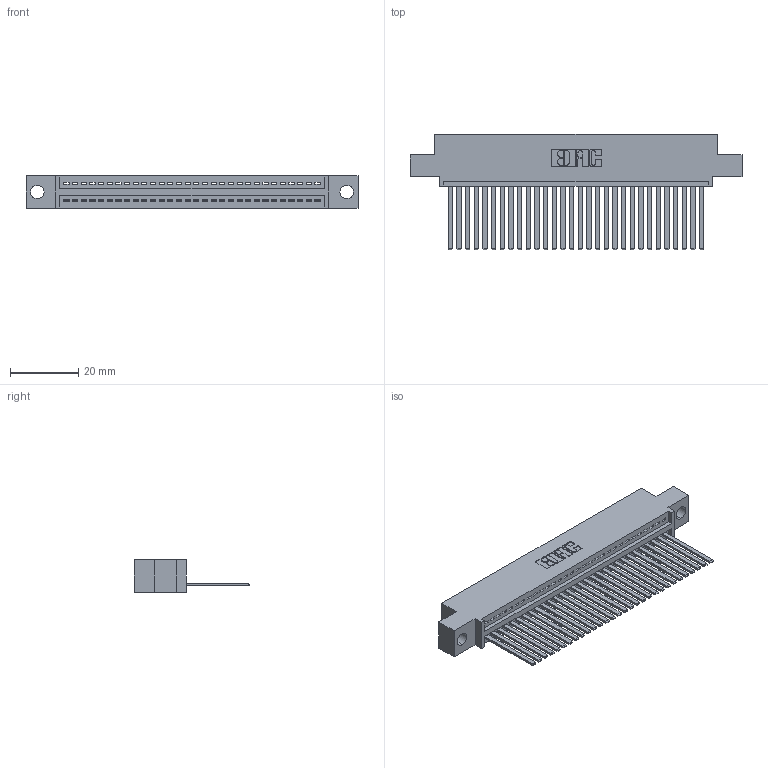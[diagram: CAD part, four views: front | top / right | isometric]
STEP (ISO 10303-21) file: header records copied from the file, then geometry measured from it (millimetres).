
FILE_DESCRIPTION (( 'STEP AP203' ), '1' );
FILE_NAME ('345-030-544-404.STEP', '2018-08-23T06:50:27', ( '' ), ( '' ), 'SwSTEP 2.0', 'SolidWorks 2016', '' );
FILE_SCHEMA (( 'CONFIG_CONTROL_DESIGN' ));
Length unit declared in the file: inch
Products named in the file (3): 345 Part_0.110 Offset - 0.156 Dia-TH; 345-292-001_345-293-144; 345-030-544-404
Assembly tree (31 placements, depth 2):
  345-030-544-404
    345 Part_0.110 Offset - 0.156 Dia-TH
    345-292-001_345-293-144  x30
Bounding box: 97.41 x 33.96 x 9.4 mm (x, y, z)
Volume: 9339.9 mm3; surface area: 13182.5 mm2
Topology: 31 solids, 31 shells, 1690 faces, 5093 edges, 3354 vertices
Faces by surface type: plane 1164, cylinder 526
Entity records: 24145 total; most frequent: CARTESIAN_POINT 4190, ORIENTED_EDGE 4154, DIRECTION 3673, EDGE_CURVE 2077, LINE 1829, VECTOR 1829, VERTEX_POINT 1382, AXIS2_PLACEMENT_3D 922
